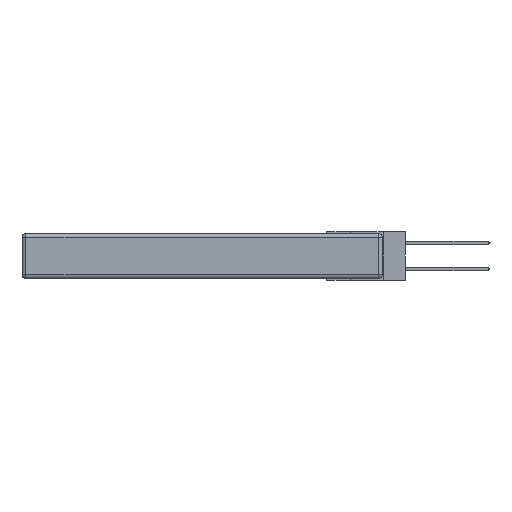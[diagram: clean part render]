
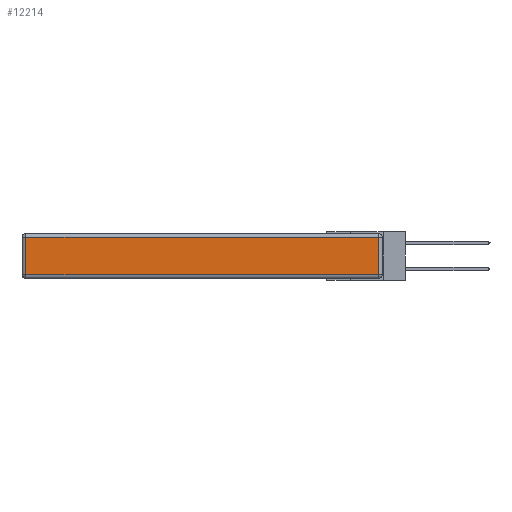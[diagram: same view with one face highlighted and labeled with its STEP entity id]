
A CAD part, left-side view. The second image highlights one B-rep face of the part: STEP entity #12214.
In plain terms, the highlighted planar face has unit normal (-1, 0, 0).
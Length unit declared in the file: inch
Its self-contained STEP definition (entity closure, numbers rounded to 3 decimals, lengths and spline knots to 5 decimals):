
#361 = DIRECTION ( 'NONE',  ( 0., 0., 1. ) ) ;
#715 = VERTEX_POINT ( 'NONE', #11630 ) ;
#1009 = CARTESIAN_POINT ( 'NONE',  ( 0., 0., -0.313 ) ) ;
#1120 = ORIENTED_EDGE ( 'NONE', *, *, #3410, .T. ) ;
#1436 = CARTESIAN_POINT ( 'NONE',  ( 0., 2.72, -0.343 ) ) ;
#1437 = DIRECTION ( 'NONE',  ( 0., 0., 1. ) ) ;
#1621 = VERTEX_POINT ( 'NONE', #18253 ) ;
#1693 = EDGE_CURVE ( 'NONE', #10324, #1621, #16962, .T. ) ;
#2514 = ORIENTED_EDGE ( 'NONE', *, *, #11387, .T. ) ;
#3410 = EDGE_CURVE ( 'NONE', #715, #10324, #16457, .T. ) ;
#5304 = CARTESIAN_POINT ( 'NONE',  ( 0., 0.03, -0.313 ) ) ;
#7027 = ORIENTED_EDGE ( 'NONE', *, *, #1693, .T. ) ;
#7150 = ORIENTED_EDGE ( 'NONE', *, *, #9922, .T. ) ;
#7370 = CARTESIAN_POINT ( 'NONE',  ( 0., 0., -0.343 ) ) ;
#7555 = PLANE ( 'NONE',  #9875 ) ;
#8050 = CARTESIAN_POINT ( 'NONE',  ( 0., 2.75, -0.03 ) ) ;
#8282 = VECTOR ( 'NONE', #14349, 39.37008 ) ;
#9009 = DIRECTION ( 'NONE',  ( -1., 0., 0. ) ) ;
#9135 = VECTOR ( 'NONE', #1437, 39.37008 ) ;
#9504 = DIRECTION ( 'NONE',  ( 0., 1., 0. ) ) ;
#9875 = AXIS2_PLACEMENT_3D ( 'NONE', #7370, #9009, #361 ) ;
#9922 = EDGE_CURVE ( 'NONE', #1621, #10151, #13468, .T. ) ;
#10073 = CARTESIAN_POINT ( 'NONE',  ( 0., 0.03, -0.343 ) ) ;
#10151 = VERTEX_POINT ( 'NONE', #5304 ) ;
#10324 = VERTEX_POINT ( 'NONE', #12567 ) ;
#11387 = EDGE_CURVE ( 'NONE', #10151, #715, #12507, .T. ) ;
#11630 = CARTESIAN_POINT ( 'NONE',  ( 0., 0.03, -0.03 ) ) ;
#12214 = ADVANCED_FACE ( 'NONE', ( #16604 ), #7555, .T. ) ;
#12507 = LINE ( 'NONE', #10073, #9135 ) ;
#12567 = CARTESIAN_POINT ( 'NONE',  ( 0., 2.72, -0.03 ) ) ;
#12568 = VECTOR ( 'NONE', #9504, 39.37008 ) ;
#13468 = LINE ( 'NONE', #1009, #8282 ) ;
#14349 = DIRECTION ( 'NONE',  ( 0., -1., 0. ) ) ;
#15129 = EDGE_LOOP ( 'NONE', ( #7150, #2514, #1120, #7027 ) ) ;
#16457 = LINE ( 'NONE', #8050, #12568 ) ;
#16604 = FACE_OUTER_BOUND ( 'NONE', #15129, .T. ) ;
#16962 = LINE ( 'NONE', #1436, #17174 ) ;
#17174 = VECTOR ( 'NONE', #17295, 39.37008 ) ;
#17295 = DIRECTION ( 'NONE',  ( 0., 0., -1. ) ) ;
#18253 = CARTESIAN_POINT ( 'NONE',  ( 0., 2.72, -0.313 ) ) ;
